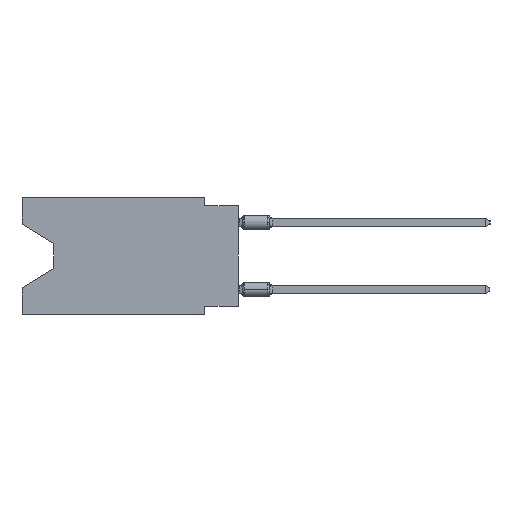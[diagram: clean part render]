
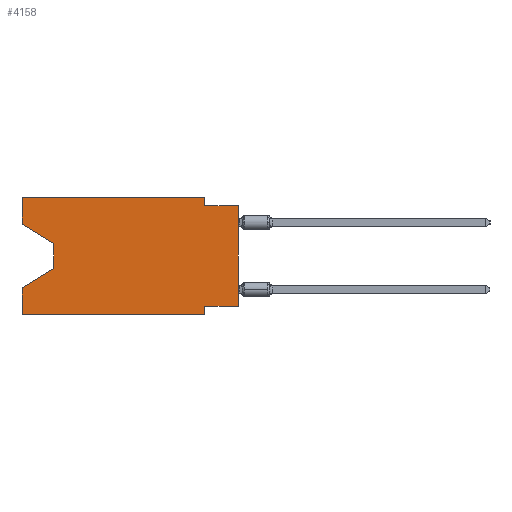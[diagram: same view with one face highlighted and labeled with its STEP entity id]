
A CAD part, left-side view. The second image highlights one B-rep face of the part: STEP entity #4158.
In plain terms, the highlighted planar face has unit normal (-1, 0, 0).
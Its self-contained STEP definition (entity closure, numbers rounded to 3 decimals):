
#408 = CARTESIAN_POINT ( 'NONE',  ( 0., 16.383, -8.89 ) ) ;
#585 = DIRECTION ( 'NONE',  ( 0., 0., -1. ) ) ;
#626 = LINE ( 'NONE', #36389, #11385 ) ;
#673 = EDGE_CURVE ( 'NONE', #26175, #27084, #11130, .T. ) ;
#1747 = LINE ( 'NONE', #27716, #28334 ) ;
#1932 = PLANE ( 'NONE',  #38036 ) ;
#2159 = DIRECTION ( 'NONE',  ( 0., -0.855, -0.519 ) ) ;
#2254 = LINE ( 'NONE', #25683, #26795 ) ;
#2410 = VECTOR ( 'NONE', #10401, 1000. ) ;
#2774 = ORIENTED_EDGE ( 'NONE', *, *, #13789, .F. ) ;
#2942 = VECTOR ( 'NONE', #18145, 1000. ) ;
#3207 = CARTESIAN_POINT ( 'NONE',  ( 0., 0., -8.255 ) ) ;
#3652 = CARTESIAN_POINT ( 'NONE',  ( 0., 0., -0.635 ) ) ;
#4022 = CARTESIAN_POINT ( 'NONE',  ( 0., 0., -0.635 ) ) ;
#4158 = ADVANCED_FACE ( 'NONE', ( #34896 ), #1932, .F. ) ;
#4444 = EDGE_CURVE ( 'NONE', #40322, #27470, #13998, .T. ) ;
#5125 = CARTESIAN_POINT ( 'NONE',  ( 0., 16.383, 0. ) ) ;
#5368 = VERTEX_POINT ( 'NONE', #40232 ) ;
#6394 = VERTEX_POINT ( 'NONE', #35341 ) ;
#6935 = CARTESIAN_POINT ( 'NONE',  ( 0., 0., -8.255 ) ) ;
#8133 = VECTOR ( 'NONE', #14401, 1000. ) ;
#9380 = EDGE_CURVE ( 'NONE', #30649, #27084, #26785, .T. ) ;
#9457 = ORIENTED_EDGE ( 'NONE', *, *, #20725, .F. ) ;
#9572 = CARTESIAN_POINT ( 'NONE',  ( 0., 16.383, 0. ) ) ;
#9601 = ORIENTED_EDGE ( 'NONE', *, *, #27414, .F. ) ;
#10167 = CARTESIAN_POINT ( 'NONE',  ( 0., 2.54, 0. ) ) ;
#10401 = DIRECTION ( 'NONE',  ( 0., 1., 0. ) ) ;
#11130 = LINE ( 'NONE', #27528, #39967 ) ;
#11385 = VECTOR ( 'NONE', #20003, 1000. ) ;
#12703 = EDGE_CURVE ( 'NONE', #36283, #6394, #1747, .T. ) ;
#13386 = VERTEX_POINT ( 'NONE', #29769 ) ;
#13706 = CARTESIAN_POINT ( 'NONE',  ( 0., 2.54, 0. ) ) ;
#13786 = LINE ( 'NONE', #3207, #2410 ) ;
#13789 = EDGE_CURVE ( 'NONE', #36034, #35115, #33318, .T. ) ;
#13998 = LINE ( 'NONE', #33806, #8133 ) ;
#14401 = DIRECTION ( 'NONE',  ( 0., -1., 0. ) ) ;
#15234 = DIRECTION ( 'NONE',  ( 0., 0., 1. ) ) ;
#15983 = EDGE_CURVE ( 'NONE', #24766, #13386, #24107, .T. ) ;
#16307 = CARTESIAN_POINT ( 'NONE',  ( 0., 16.383, 0. ) ) ;
#16595 = CARTESIAN_POINT ( 'NONE',  ( 0., 2.54, -8.89 ) ) ;
#16811 = DIRECTION ( 'NONE',  ( 0., -1., 0. ) ) ;
#17074 = EDGE_CURVE ( 'NONE', #40322, #13386, #2254, .T. ) ;
#17127 = DIRECTION ( 'NONE',  ( 0., 0., 1. ) ) ;
#17220 = CARTESIAN_POINT ( 'NONE',  ( 0., 13.97, -3.505 ) ) ;
#18145 = DIRECTION ( 'NONE',  ( 0., 0.855, -0.519 ) ) ;
#19172 = EDGE_LOOP ( 'NONE', ( #35473, #37753, #34526, #25198, #21164, #9457, #9601, #30068, #34668, #26389, #2774, #24250 ) ) ;
#19421 = VECTOR ( 'NONE', #39296, 1000. ) ;
#19917 = CARTESIAN_POINT ( 'NONE',  ( 0., 16.383, 0. ) ) ;
#20003 = DIRECTION ( 'NONE',  ( 0., 0., -1. ) ) ;
#20725 = EDGE_CURVE ( 'NONE', #5368, #27470, #626, .T. ) ;
#21164 = ORIENTED_EDGE ( 'NONE', *, *, #4444, .T. ) ;
#21477 = EDGE_CURVE ( 'NONE', #36283, #36034, #29904, .T. ) ;
#21522 = VECTOR ( 'NONE', #39172, 1000. ) ;
#21854 = CARTESIAN_POINT ( 'NONE',  ( 0., 16.383, -2.038 ) ) ;
#21870 = CARTESIAN_POINT ( 'NONE',  ( 0., 13.97, -5.385 ) ) ;
#24107 = LINE ( 'NONE', #28127, #2942 ) ;
#24136 = VECTOR ( 'NONE', #16811, 1000. ) ;
#24250 = ORIENTED_EDGE ( 'NONE', *, *, #21477, .F. ) ;
#24552 = EDGE_CURVE ( 'NONE', #6394, #24766, #39788, .T. ) ;
#24766 = VERTEX_POINT ( 'NONE', #21870 ) ;
#25123 = DIRECTION ( 'NONE',  ( 0., 0., -1. ) ) ;
#25198 = ORIENTED_EDGE ( 'NONE', *, *, #17074, .F. ) ;
#25683 = CARTESIAN_POINT ( 'NONE',  ( 0., 16.383, 0. ) ) ;
#26175 = VERTEX_POINT ( 'NONE', #6935 ) ;
#26389 = ORIENTED_EDGE ( 'NONE', *, *, #34590, .F. ) ;
#26785 = LINE ( 'NONE', #4022, #24136 ) ;
#26795 = VECTOR ( 'NONE', #15234, 1000. ) ;
#27084 = VERTEX_POINT ( 'NONE', #3652 ) ;
#27414 = EDGE_CURVE ( 'NONE', #26175, #5368, #13786, .T. ) ;
#27470 = VERTEX_POINT ( 'NONE', #16595 ) ;
#27528 = CARTESIAN_POINT ( 'NONE',  ( 0., 0., 0. ) ) ;
#27716 = CARTESIAN_POINT ( 'NONE',  ( 0., 16.383, -2.038 ) ) ;
#27951 = CARTESIAN_POINT ( 'NONE',  ( 0., 2.54, -0.635 ) ) ;
#28127 = CARTESIAN_POINT ( 'NONE',  ( 0., 13.97, -5.385 ) ) ;
#28334 = VECTOR ( 'NONE', #2159, 1000. ) ;
#29769 = CARTESIAN_POINT ( 'NONE',  ( 0., 16.383, -6.852 ) ) ;
#29904 = LINE ( 'NONE', #16307, #33189 ) ;
#30068 = ORIENTED_EDGE ( 'NONE', *, *, #673, .T. ) ;
#30515 = DIRECTION ( 'NONE',  ( 0., 0., 1. ) ) ;
#30649 = VERTEX_POINT ( 'NONE', #27951 ) ;
#32544 = LINE ( 'NONE', #10167, #34934 ) ;
#33189 = VECTOR ( 'NONE', #17127, 1000. ) ;
#33318 = LINE ( 'NONE', #19917, #19421 ) ;
#33806 = CARTESIAN_POINT ( 'NONE',  ( 0., 16.383, -8.89 ) ) ;
#34526 = ORIENTED_EDGE ( 'NONE', *, *, #15983, .T. ) ;
#34590 = EDGE_CURVE ( 'NONE', #35115, #30649, #32544, .T. ) ;
#34668 = ORIENTED_EDGE ( 'NONE', *, *, #9380, .F. ) ;
#34896 = FACE_OUTER_BOUND ( 'NONE', #19172, .T. ) ;
#34934 = VECTOR ( 'NONE', #585, 1000. ) ;
#35115 = VERTEX_POINT ( 'NONE', #13706 ) ;
#35341 = CARTESIAN_POINT ( 'NONE',  ( 0., 13.97, -3.505 ) ) ;
#35473 = ORIENTED_EDGE ( 'NONE', *, *, #12703, .T. ) ;
#36034 = VERTEX_POINT ( 'NONE', #9572 ) ;
#36283 = VERTEX_POINT ( 'NONE', #21854 ) ;
#36389 = CARTESIAN_POINT ( 'NONE',  ( 0., 2.54, -8.89 ) ) ;
#37753 = ORIENTED_EDGE ( 'NONE', *, *, #24552, .T. ) ;
#38036 = AXIS2_PLACEMENT_3D ( 'NONE', #5125, #40662, #25123 ) ;
#39172 = DIRECTION ( 'NONE',  ( 0., 0., -1. ) ) ;
#39296 = DIRECTION ( 'NONE',  ( 0., -1., 0. ) ) ;
#39788 = LINE ( 'NONE', #17220, #21522 ) ;
#39967 = VECTOR ( 'NONE', #30515, 1000. ) ;
#40232 = CARTESIAN_POINT ( 'NONE',  ( 0., 2.54, -8.255 ) ) ;
#40322 = VERTEX_POINT ( 'NONE', #408 ) ;
#40662 = DIRECTION ( 'NONE',  ( 1., 0., 0. ) ) ;
